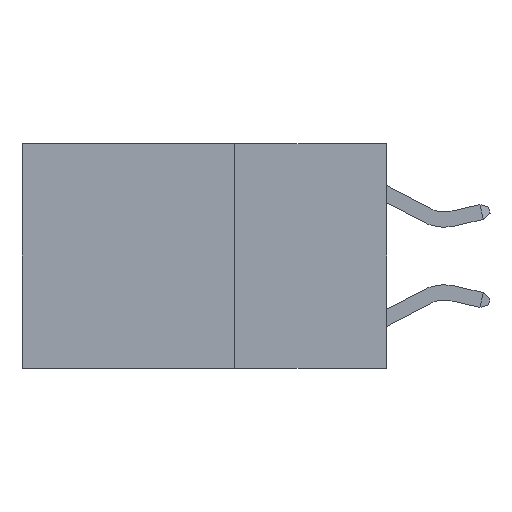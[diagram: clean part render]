
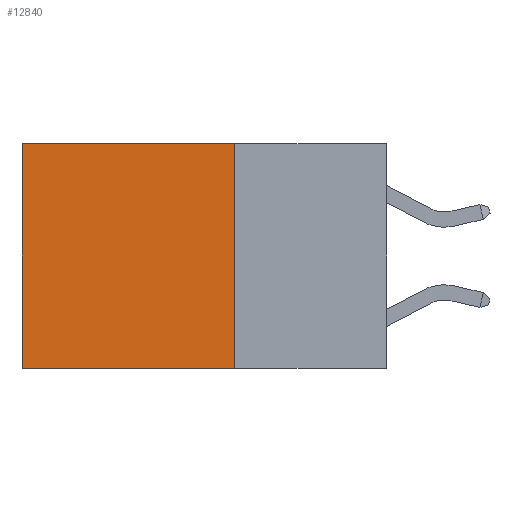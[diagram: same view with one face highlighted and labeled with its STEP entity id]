
A CAD part, left-side view. The second image highlights one B-rep face of the part: STEP entity #12840.
In plain terms, the highlighted planar face has unit normal (-1, 0, 0).
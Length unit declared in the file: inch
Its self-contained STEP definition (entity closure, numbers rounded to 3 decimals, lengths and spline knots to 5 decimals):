
#565 = ORIENTED_EDGE ( 'NONE', *, *, #2863, .T. ) ;
#592 = LINE ( 'NONE', #2623, #16738 ) ;
#780 = DIRECTION ( 'NONE',  ( 0., 0., -1. ) ) ;
#1544 = CARTESIAN_POINT ( 'NONE',  ( 0.2625, 0.25, 0. ) ) ;
#1805 = ORIENTED_EDGE ( 'NONE', *, *, #3925, .F. ) ;
#1979 = DIRECTION ( 'NONE',  ( 0., 1., 0. ) ) ;
#2355 = ORIENTED_EDGE ( 'NONE', *, *, #16098, .F. ) ;
#2623 = CARTESIAN_POINT ( 'NONE',  ( 0.2625, 0.25, 0. ) ) ;
#2863 = EDGE_CURVE ( 'NONE', #10281, #15733, #592, .T. ) ;
#2921 = DIRECTION ( 'NONE',  ( 1., 0., 0. ) ) ;
#3567 = LINE ( 'NONE', #14773, #4204 ) ;
#3925 = EDGE_CURVE ( 'NONE', #10281, #11458, #3567, .T. ) ;
#4204 = VECTOR ( 'NONE', #780, 39.37008 ) ;
#6020 = VECTOR ( 'NONE', #15520, 39.37008 ) ;
#7801 = CARTESIAN_POINT ( 'NONE',  ( 0.2625, 0.6, -0.37 ) ) ;
#7876 = AXIS2_PLACEMENT_3D ( 'NONE', #1544, #2921, #12511 ) ;
#8356 = LINE ( 'NONE', #11659, #12449 ) ;
#9704 = CARTESIAN_POINT ( 'NONE',  ( 0.2625, 0.6, 0. ) ) ;
#9942 = FACE_OUTER_BOUND ( 'NONE', #16417, .T. ) ;
#10281 = VERTEX_POINT ( 'NONE', #16929 ) ;
#11038 = DIRECTION ( 'NONE',  ( 0., 1., 0. ) ) ;
#11371 = EDGE_CURVE ( 'NONE', #15733, #14503, #13765, .T. ) ;
#11458 = VERTEX_POINT ( 'NONE', #13026 ) ;
#11659 = CARTESIAN_POINT ( 'NONE',  ( 0.2625, 0.25, -0.37 ) ) ;
#11770 = ORIENTED_EDGE ( 'NONE', *, *, #11371, .T. ) ;
#12449 = VECTOR ( 'NONE', #1979, 39.37008 ) ;
#12511 = DIRECTION ( 'NONE',  ( 0., 0., -1. ) ) ;
#12840 = ADVANCED_FACE ( 'NONE', ( #9942 ), #16507, .F. ) ;
#13026 = CARTESIAN_POINT ( 'NONE',  ( 0.2625, 0.25, -0.37 ) ) ;
#13765 = LINE ( 'NONE', #17075, #6020 ) ;
#14503 = VERTEX_POINT ( 'NONE', #7801 ) ;
#14773 = CARTESIAN_POINT ( 'NONE',  ( 0.2625, 0.25, 0. ) ) ;
#15520 = DIRECTION ( 'NONE',  ( 0., 0., -1. ) ) ;
#15733 = VERTEX_POINT ( 'NONE', #9704 ) ;
#16098 = EDGE_CURVE ( 'NONE', #11458, #14503, #8356, .T. ) ;
#16417 = EDGE_LOOP ( 'NONE', ( #11770, #2355, #1805, #565 ) ) ;
#16507 = PLANE ( 'NONE',  #7876 ) ;
#16738 = VECTOR ( 'NONE', #11038, 39.37008 ) ;
#16929 = CARTESIAN_POINT ( 'NONE',  ( 0.2625, 0.25, 0. ) ) ;
#17075 = CARTESIAN_POINT ( 'NONE',  ( 0.2625, 0.6, 0. ) ) ;
